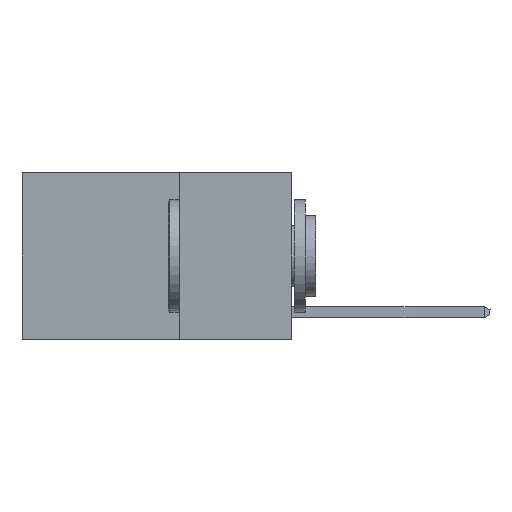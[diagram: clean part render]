
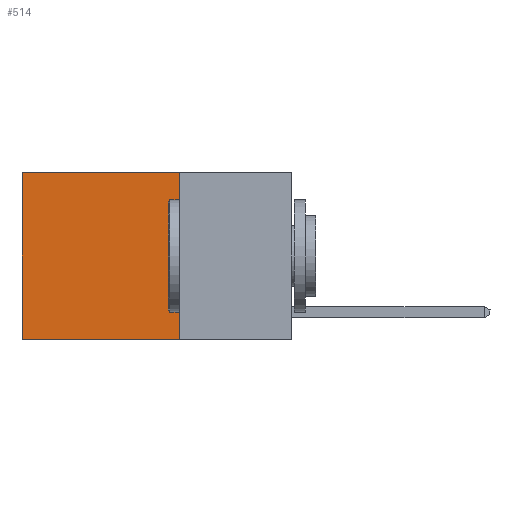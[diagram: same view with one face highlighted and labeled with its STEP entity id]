
A CAD part, left-side view. The second image highlights one B-rep face of the part: STEP entity #514.
In plain terms, the highlighted planar face has unit normal (-1, 0, 0).
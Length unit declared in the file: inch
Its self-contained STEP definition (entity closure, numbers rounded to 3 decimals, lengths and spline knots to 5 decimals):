
#40 = CARTESIAN_POINT ( 'NONE',  ( 0.2625, 0.6, 0. ) ) ;
#185 = VECTOR ( 'NONE', #2057, 39.37008 ) ;
#514 = ADVANCED_FACE ( 'NONE', ( #8100 ), #8780, .F. ) ;
#589 = ORIENTED_EDGE ( 'NONE', *, *, #2914, .F. ) ;
#877 = ORIENTED_EDGE ( 'NONE', *, *, #10076, .T. ) ;
#2057 = DIRECTION ( 'NONE',  ( 0., 0., -1. ) ) ;
#2376 = ORIENTED_EDGE ( 'NONE', *, *, #5204, .T. ) ;
#2576 = CARTESIAN_POINT ( 'NONE',  ( 0.2625, 0.6, 0. ) ) ;
#2687 = VERTEX_POINT ( 'NONE', #7335 ) ;
#2740 = ORIENTED_EDGE ( 'NONE', *, *, #2824, .F. ) ;
#2824 = EDGE_CURVE ( 'NONE', #10675, #2687, #4807, .T. ) ;
#2914 = EDGE_CURVE ( 'NONE', #2687, #7170, #10141, .T. ) ;
#4421 = CARTESIAN_POINT ( 'NONE',  ( 0.2625, 0.25, 0. ) ) ;
#4633 = LINE ( 'NONE', #6719, #8138 ) ;
#4807 = LINE ( 'NONE', #8670, #185 ) ;
#5022 = DIRECTION ( 'NONE',  ( 0., 0., -1. ) ) ;
#5204 = EDGE_CURVE ( 'NONE', #10675, #9337, #4633, .T. ) ;
#5353 = EDGE_LOOP ( 'NONE', ( #877, #589, #2740, #2376 ) ) ;
#5513 = DIRECTION ( 'NONE',  ( 0., 1., 0. ) ) ;
#6250 = LINE ( 'NONE', #2576, #8172 ) ;
#6508 = VECTOR ( 'NONE', #5513, 39.37008 ) ;
#6582 = CARTESIAN_POINT ( 'NONE',  ( 0.2625, 0.6, -0.37 ) ) ;
#6719 = CARTESIAN_POINT ( 'NONE',  ( 0.2625, 0.25, 0. ) ) ;
#6987 = DIRECTION ( 'NONE',  ( 1., 0., 0. ) ) ;
#7170 = VERTEX_POINT ( 'NONE', #6582 ) ;
#7335 = CARTESIAN_POINT ( 'NONE',  ( 0.2625, 0.25, -0.37 ) ) ;
#7811 = DIRECTION ( 'NONE',  ( 0., 0., -1. ) ) ;
#7980 = CARTESIAN_POINT ( 'NONE',  ( 0.2625, 0.25, -0.37 ) ) ;
#8100 = FACE_OUTER_BOUND ( 'NONE', #5353, .T. ) ;
#8138 = VECTOR ( 'NONE', #10140, 39.37008 ) ;
#8172 = VECTOR ( 'NONE', #5022, 39.37008 ) ;
#8626 = AXIS2_PLACEMENT_3D ( 'NONE', #9438, #6987, #7811 ) ;
#8670 = CARTESIAN_POINT ( 'NONE',  ( 0.2625, 0.25, 0. ) ) ;
#8780 = PLANE ( 'NONE',  #8626 ) ;
#9337 = VERTEX_POINT ( 'NONE', #40 ) ;
#9438 = CARTESIAN_POINT ( 'NONE',  ( 0.2625, 0.25, 0. ) ) ;
#10076 = EDGE_CURVE ( 'NONE', #9337, #7170, #6250, .T. ) ;
#10140 = DIRECTION ( 'NONE',  ( 0., 1., 0. ) ) ;
#10141 = LINE ( 'NONE', #7980, #6508 ) ;
#10675 = VERTEX_POINT ( 'NONE', #4421 ) ;
